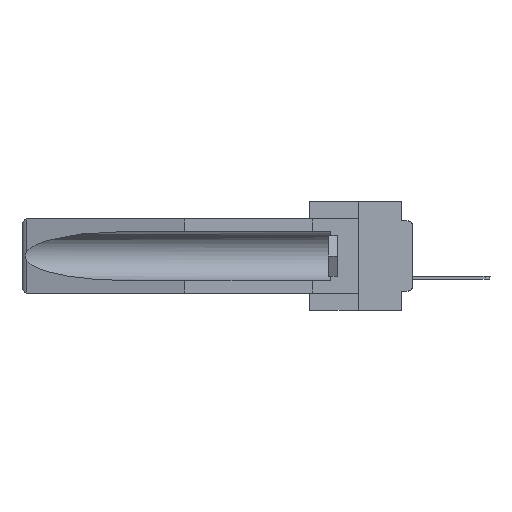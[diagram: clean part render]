
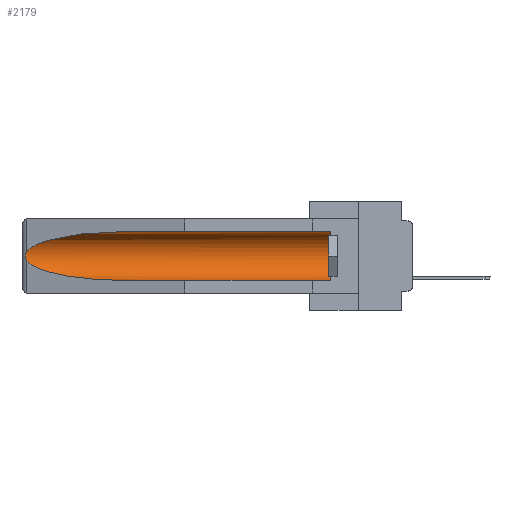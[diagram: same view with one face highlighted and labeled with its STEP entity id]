
A CAD part, left-side view. The second image highlights one B-rep face of the part: STEP entity #2179.
In plain terms, the highlighted cylindrical face has radius 2.857 mm (diameter 5.715 mm), a partial arc.
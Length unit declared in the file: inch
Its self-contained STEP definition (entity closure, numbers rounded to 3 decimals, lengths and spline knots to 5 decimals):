
#86 = CARTESIAN_POINT ( 'NONE',  ( 0.2673, 1.53269, -0.17917 ) ) ;
#665 = CARTESIAN_POINT ( 'NONE',  ( 0.26597, 1.5296, -0.19026 ) ) ;
#696 = B_SPLINE_CURVE_WITH_KNOTS ( 'NONE', 3,
 ( #32141, #12121, #35180, #35554, #28898, #8670, #86, #26028, #665, #8867 ),
 .UNSPECIFIED., .F., .F.,
 ( 4, 2, 2, 2, 4 ),
 ( 0., 0.00029, 0.00058, 0.00087, 0.00117 ),
 .UNSPECIFIED. ) ;
#1292 = EDGE_CURVE ( 'NONE', #4019, #9800, #696, .T. ) ;
#2179 = ADVANCED_FACE ( 'NONE', ( #11017 ), #22657, .F. ) ;
#2407 = AXIS2_PLACEMENT_3D ( 'NONE', #2612, #37514, #34265 ) ;
#2592 = CARTESIAN_POINT ( 'NONE',  ( 0.26537, 1.52718, -0.19328 ) ) ;
#2612 = CARTESIAN_POINT ( 'NONE',  ( 0.155, -0.30754, -0.1715 ) ) ;
#2871 = EDGE_CURVE ( 'NONE', #3867, #4019, #27274, .T. ) ;
#3475 = AXIS2_PLACEMENT_3D ( 'NONE', #31903, #17232, #29415 ) ;
#3867 = VERTEX_POINT ( 'NONE', #16727 ) ;
#4019 = VERTEX_POINT ( 'NONE', #37667 ) ;
#4176 = LINE ( 'NONE', #20968, #32462 ) ;
#4234 = CARTESIAN_POINT ( 'NONE',  ( 0.155, 1.07973, -0.059 ) ) ;
#4386 = ORIENTED_EDGE ( 'NONE', *, *, #18263, .T. ) ;
#4871 = LINE ( 'NONE', #5045, #19324 ) ;
#5045 = CARTESIAN_POINT ( 'NONE',  ( 0.155, -0.30754, -0.284 ) ) ;
#5470 = CARTESIAN_POINT ( 'NONE',  ( 0.155, 1.07973, -0.284 ) ) ;
#6784 = VERTEX_POINT ( 'NONE', #9350 ) ;
#8670 = CARTESIAN_POINT ( 'NONE',  ( 0.2675, 1.53308, -0.17534 ) ) ;
#8867 = CARTESIAN_POINT ( 'NONE',  ( 0.26537, 1.52718, -0.19328 ) ) ;
#9350 = CARTESIAN_POINT ( 'NONE',  ( 0.155, 0.126, -0.284 ) ) ;
#9800 = VERTEX_POINT ( 'NONE', #9886 ) ;
#9886 = CARTESIAN_POINT ( 'NONE',  ( 0.26537, 1.52718, -0.19328 ) ) ;
#10174 = CIRCLE ( 'NONE', #3475, 0.1125 ) ;
#10326 = ORIENTED_EDGE ( 'NONE', *, *, #30515, .F. ) ;
#10407 = DIRECTION ( 'NONE',  ( 0., 1., 0. ) ) ;
#11017 = FACE_OUTER_BOUND ( 'NONE', #13082, .T. ) ;
#11568 = CARTESIAN_POINT ( 'NONE',  ( 0.21114, 1.30732, -0.284 ) ) ;
#12121 = CARTESIAN_POINT ( 'NONE',  ( 0.26597, 1.52961, -0.15275 ) ) ;
#13007 = CARTESIAN_POINT ( 'NONE',  ( 0.25451, 1.48313, -0.09465 ) ) ;
#13082 = EDGE_LOOP ( 'NONE', ( #36000, #13291, #20747, #10326, #4386, #31209 ) ) ;
#13291 = ORIENTED_EDGE ( 'NONE', *, *, #1292, .T. ) ;
#15147 = VERTEX_POINT ( 'NONE', #16156 ) ;
#15827 = DIRECTION ( 'NONE',  ( 0., 1., 0. ) ) ;
#15882 = CARTESIAN_POINT ( 'NONE',  ( 0.21114, 1.30732, -0.059 ) ) ;
#16156 = CARTESIAN_POINT ( 'NONE',  ( 0.155, 0.126, -0.059 ) ) ;
#16727 = CARTESIAN_POINT ( 'NONE',  ( 0.155, 1.07973, -0.059 ) ) ;
#17232 = DIRECTION ( 'NONE',  ( 0., -1., 0. ) ) ;
#17940 = EDGE_CURVE ( 'NONE', #15147, #3867, #4176, .T. ) ;
#18263 = EDGE_CURVE ( 'NONE', #6784, #15147, #10174, .T. ) ;
#19324 = VECTOR ( 'NONE', #10407, 39.37008 ) ;
#20747 = ORIENTED_EDGE ( 'NONE', *, *, #21264, .T. ) ;
#20968 = CARTESIAN_POINT ( 'NONE',  ( 0.155, -0.30754, -0.059 ) ) ;
#21264 = EDGE_CURVE ( 'NONE', #9800, #25501, #35058, .T. ) ;
#22272 = CARTESIAN_POINT ( 'NONE',  ( 0.155, 1.07973, -0.284 ) ) ;
#22348 = CARTESIAN_POINT ( 'NONE',  ( 0.26537, 1.52718, -0.14972 ) ) ;
#22657 = CYLINDRICAL_SURFACE ( 'NONE', #2407, 0.1125 ) ;
#25501 = VERTEX_POINT ( 'NONE', #22272 ) ;
#26028 = CARTESIAN_POINT ( 'NONE',  ( 0.26655, 1.53094, -0.18657 ) ) ;
#27274 =( BOUNDED_CURVE ( )  B_SPLINE_CURVE ( 3, ( #4234, #15882, #13007, #22348 ),
 .UNSPECIFIED., .F., .F. ) 
 B_SPLINE_CURVE_WITH_KNOTS ( ( 4, 4 ),
 ( 4.71239, 6.08839 ),
 .UNSPECIFIED. ) 
 CURVE ( )  GEOMETRIC_REPRESENTATION_ITEM ( )  RATIONAL_B_SPLINE_CURVE ( ( 1., 0.848, 0.848, 1. ) ) 
 REPRESENTATION_ITEM ( '' )  );
#28898 = CARTESIAN_POINT ( 'NONE',  ( 0.2675, 1.53308, -0.16763 ) ) ;
#29415 = DIRECTION ( 'NONE',  ( 0., 0., 1. ) ) ;
#30515 = EDGE_CURVE ( 'NONE', #6784, #25501, #4871, .T. ) ;
#31209 = ORIENTED_EDGE ( 'NONE', *, *, #17940, .T. ) ;
#31903 = CARTESIAN_POINT ( 'NONE',  ( 0.155, 0.126, -0.1715 ) ) ;
#32141 = CARTESIAN_POINT ( 'NONE',  ( 0.26537, 1.52718, -0.14972 ) ) ;
#32462 = VECTOR ( 'NONE', #15827, 39.37008 ) ;
#34249 = CARTESIAN_POINT ( 'NONE',  ( 0.25451, 1.48313, -0.24835 ) ) ;
#34265 = DIRECTION ( 'NONE',  ( 0., 0., 1. ) ) ;
#35058 =( BOUNDED_CURVE ( )  B_SPLINE_CURVE ( 3, ( #2592, #34249, #11568, #5470 ),
 .UNSPECIFIED., .F., .F. ) 
 B_SPLINE_CURVE_WITH_KNOTS ( ( 4, 4 ),
 ( 0.1948, 1.5708 ),
 .UNSPECIFIED. ) 
 CURVE ( )  GEOMETRIC_REPRESENTATION_ITEM ( )  RATIONAL_B_SPLINE_CURVE ( ( 1., 0.848, 0.848, 1. ) ) 
 REPRESENTATION_ITEM ( '' )  );
#35180 = CARTESIAN_POINT ( 'NONE',  ( 0.26654, 1.53092, -0.15636 ) ) ;
#35554 = CARTESIAN_POINT ( 'NONE',  ( 0.2673, 1.5327, -0.16383 ) ) ;
#36000 = ORIENTED_EDGE ( 'NONE', *, *, #2871, .T. ) ;
#37514 = DIRECTION ( 'NONE',  ( 0., 1., 0. ) ) ;
#37667 = CARTESIAN_POINT ( 'NONE',  ( 0.26537, 1.52718, -0.14972 ) ) ;
